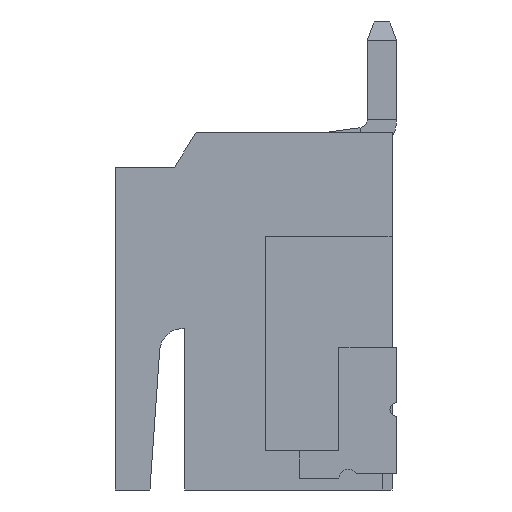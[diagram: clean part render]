
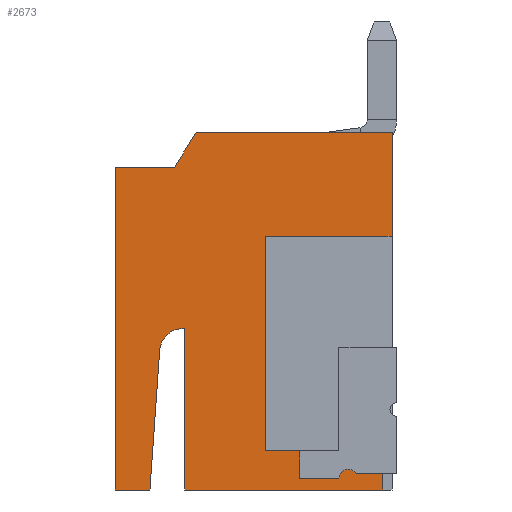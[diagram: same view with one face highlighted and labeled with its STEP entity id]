
A CAD part, left-side view. The second image highlights one B-rep face of the part: STEP entity #2673.
In plain terms, the highlighted planar face has unit normal (-1, 0, 0).
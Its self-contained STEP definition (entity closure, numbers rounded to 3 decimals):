
#42 = DIRECTION ( 'NONE',  ( 0., 0., 1. ) ) ;
#72 = DIRECTION ( 'NONE',  ( 0., 0., -1. ) ) ;
#179 = EDGE_CURVE ( 'NONE', #2912, #4283, #1416, .T. ) ;
#268 = LINE ( 'NONE', #2807, #2163 ) ;
#281 = CARTESIAN_POINT ( 'NONE',  ( -6.25, -3.1, 3.875 ) ) ;
#428 = DIRECTION ( 'NONE',  ( 0., 0., 1. ) ) ;
#491 = CARTESIAN_POINT ( 'NONE',  ( -6.25, 1.619, 3.125 ) ) ;
#529 = CARTESIAN_POINT ( 'NONE',  ( -6.25, -2.9, 3.875 ) ) ;
#533 = CARTESIAN_POINT ( 'NONE',  ( -6.25, -2.9, -3.525 ) ) ;
#568 = VECTOR ( 'NONE', #6327, 1000. ) ;
#625 = LINE ( 'NONE', #2637, #4047 ) ;
#631 = CARTESIAN_POINT ( 'NONE',  ( -6.25, 1.87, 0.131 ) ) ;
#666 = ORIENTED_EDGE ( 'NONE', *, *, #1401, .T. ) ;
#697 = EDGE_CURVE ( 'NONE', #4283, #6378, #1847, .T. ) ;
#701 = CARTESIAN_POINT ( 'NONE',  ( -6.25, -2.15, -3.625 ) ) ;
#812 = EDGE_CURVE ( 'NONE', #3117, #1203, #4040, .T. ) ;
#851 = DIRECTION ( 'NONE',  ( 0., 1., 0. ) ) ;
#862 = AXIS2_PLACEMENT_3D ( 'NONE', #4257, #6275, #2281 ) ;
#914 = ORIENTED_EDGE ( 'NONE', *, *, #1289, .T. ) ;
#956 = DIRECTION ( 'NONE',  ( 0., 1., 0. ) ) ;
#1022 = CARTESIAN_POINT ( 'NONE',  ( -6.25, -0.35, 1.625 ) ) ;
#1098 = CARTESIAN_POINT ( 'NONE',  ( -6.25, -2.323, -3.525 ) ) ;
#1147 = ORIENTED_EDGE ( 'NONE', *, *, #5128, .T. ) ;
#1203 = VERTEX_POINT ( 'NONE', #2487 ) ;
#1289 = EDGE_CURVE ( 'NONE', #4978, #3504, #3168, .T. ) ;
#1334 = CARTESIAN_POINT ( 'NONE',  ( -6.25, -0.35, 1.625 ) ) ;
#1401 = EDGE_CURVE ( 'NONE', #1934, #2912, #5885, .T. ) ;
#1416 = LINE ( 'NONE', #2936, #2177 ) ;
#1480 = CARTESIAN_POINT ( 'NONE',  ( -6.25, 1.439, -0.873 ) ) ;
#1496 = ORIENTED_EDGE ( 'NONE', *, *, #6158, .F. ) ;
#1528 = VECTOR ( 'NONE', #956, 1000. ) ;
#1649 = LINE ( 'NONE', #529, #2906 ) ;
#1666 = ORIENTED_EDGE ( 'NONE', *, *, #3754, .F. ) ;
#1847 = LINE ( 'NONE', #3853, #3435 ) ;
#1856 = CARTESIAN_POINT ( 'NONE',  ( -6.25, -0.35, -3.025 ) ) ;
#1871 = DIRECTION ( 'NONE',  ( 0., 0., -1. ) ) ;
#1874 = VERTEX_POINT ( 'NONE', #2864 ) ;
#1908 = CARTESIAN_POINT ( 'NONE',  ( -6.25, 2.15, -3.875 ) ) ;
#1934 = VERTEX_POINT ( 'NONE', #3322 ) ;
#1966 = CARTESIAN_POINT ( 'NONE',  ( -6.25, 1.4, -3.875 ) ) ;
#2133 = LINE ( 'NONE', #2265, #3410 ) ;
#2143 = CARTESIAN_POINT ( 'NONE',  ( -6.25, -1.95, -3.625 ) ) ;
#2163 = VECTOR ( 'NONE', #851, 1000. ) ;
#2177 = VECTOR ( 'NONE', #2342, 1000. ) ;
#2216 = DIRECTION ( 'NONE',  ( 0., 0., -1. ) ) ;
#2247 = PLANE ( 'NONE',  #862 ) ;
#2265 = CARTESIAN_POINT ( 'NONE',  ( -6.25, 1.4, 0. ) ) ;
#2281 = DIRECTION ( 'NONE',  ( 0., 0., -1. ) ) ;
#2288 = VECTOR ( 'NONE', #4508, 1000. ) ;
#2342 = DIRECTION ( 'NONE',  ( 0., -1., 0. ) ) ;
#2443 = CARTESIAN_POINT ( 'NONE',  ( -6.25, -2.9, -3.875 ) ) ;
#2474 = VECTOR ( 'NONE', #4161, 1000. ) ;
#2487 = CARTESIAN_POINT ( 'NONE',  ( -6.25, 1.15, 3.875 ) ) ;
#2637 = CARTESIAN_POINT ( 'NONE',  ( -6.25, 1.15, 3.875 ) ) ;
#2673 = ADVANCED_FACE ( 'NONE', ( #2741 ), #2247, .F. ) ;
#2679 = ORIENTED_EDGE ( 'NONE', *, *, #2937, .T. ) ;
#2693 = CIRCLE ( 'NONE', #4911, 0.2 ) ;
#2711 = DIRECTION ( 'NONE',  ( -1., 0., 0. ) ) ;
#2733 = CIRCLE ( 'NONE', #3457, 0.5 ) ;
#2741 = FACE_OUTER_BOUND ( 'NONE', #5272, .T. ) ;
#2761 = CARTESIAN_POINT ( 'NONE',  ( -6.25, -3.1, 1.625 ) ) ;
#2807 = CARTESIAN_POINT ( 'NONE',  ( -6.25, -2.9, -3.875 ) ) ;
#2821 = DIRECTION ( 'NONE',  ( 0., -1., 0. ) ) ;
#2848 = ORIENTED_EDGE ( 'NONE', *, *, #812, .F. ) ;
#2864 = CARTESIAN_POINT ( 'NONE',  ( -6.25, 1.938, -0.839 ) ) ;
#2906 = VECTOR ( 'NONE', #6130, 1000. ) ;
#2912 = VERTEX_POINT ( 'NONE', #1022 ) ;
#2936 = CARTESIAN_POINT ( 'NONE',  ( -6.25, -2.9, 1.625 ) ) ;
#2937 = EDGE_CURVE ( 'NONE', #1874, #6040, #2733, .T. ) ;
#2954 = VERTEX_POINT ( 'NONE', #3085 ) ;
#2974 = CARTESIAN_POINT ( 'NONE',  ( -6.25, 1.4, -0.375 ) ) ;
#3073 = ORIENTED_EDGE ( 'NONE', *, *, #4205, .F. ) ;
#3085 = CARTESIAN_POINT ( 'NONE',  ( -6.25, 2.9, 3.125 ) ) ;
#3087 = DIRECTION ( 'NONE',  ( 0., -1., 0. ) ) ;
#3117 = VERTEX_POINT ( 'NONE', #4441 ) ;
#3130 = CARTESIAN_POINT ( 'NONE',  ( -6.25, 2.9, -3.875 ) ) ;
#3132 = VERTEX_POINT ( 'NONE', #1908 ) ;
#3168 = LINE ( 'NONE', #1098, #4431 ) ;
#3199 = ORIENTED_EDGE ( 'NONE', *, *, #5900, .F. ) ;
#3243 = ORIENTED_EDGE ( 'NONE', *, *, #5388, .F. ) ;
#3322 = CARTESIAN_POINT ( 'NONE',  ( -6.25, -0.35, -3.025 ) ) ;
#3410 = VECTOR ( 'NONE', #1871, 1000. ) ;
#3422 = VECTOR ( 'NONE', #42, 1000. ) ;
#3435 = VECTOR ( 'NONE', #428, 1000. ) ;
#3457 = AXIS2_PLACEMENT_3D ( 'NONE', #1480, #3486, #72 ) ;
#3486 = DIRECTION ( 'NONE',  ( 1., 0., 0. ) ) ;
#3504 = VERTEX_POINT ( 'NONE', #5168 ) ;
#3531 = ORIENTED_EDGE ( 'NONE', *, *, #179, .T. ) ;
#3579 = VECTOR ( 'NONE', #4302, 1000. ) ;
#3591 = CARTESIAN_POINT ( 'NONE',  ( -6.25, -1.1, -3.025 ) ) ;
#3684 = VERTEX_POINT ( 'NONE', #4045 ) ;
#3695 = CARTESIAN_POINT ( 'NONE',  ( -6.25, 2.9, -3.875 ) ) ;
#3754 = EDGE_CURVE ( 'NONE', #3132, #6255, #268, .T. ) ;
#3849 = VECTOR ( 'NONE', #4857, 1000. ) ;
#3853 = CARTESIAN_POINT ( 'NONE',  ( -6.25, -3.1, 3.875 ) ) ;
#3933 = ORIENTED_EDGE ( 'NONE', *, *, #4157, .T. ) ;
#4040 = LINE ( 'NONE', #491, #2288 ) ;
#4045 = CARTESIAN_POINT ( 'NONE',  ( -6.25, -1.1, -3.625 ) ) ;
#4047 = VECTOR ( 'NONE', #3087, 1000. ) ;
#4157 = EDGE_CURVE ( 'NONE', #6040, #5623, #2133, .T. ) ;
#4161 = DIRECTION ( 'NONE',  ( 0., -0.07, 0.998 ) ) ;
#4194 = LINE ( 'NONE', #3130, #3422 ) ;
#4205 = EDGE_CURVE ( 'NONE', #4726, #5623, #6260, .T. ) ;
#4257 = CARTESIAN_POINT ( 'NONE',  ( -6.25, 0., 0. ) ) ;
#4283 = VERTEX_POINT ( 'NONE', #2761 ) ;
#4302 = DIRECTION ( 'NONE',  ( 0., 0., 1. ) ) ;
#4431 = VECTOR ( 'NONE', #6141, 1000. ) ;
#4441 = CARTESIAN_POINT ( 'NONE',  ( -6.25, 1.619, 3.125 ) ) ;
#4508 = DIRECTION ( 'NONE',  ( 0., -0.53, 0.848 ) ) ;
#4726 = VERTEX_POINT ( 'NONE', #2443 ) ;
#4857 = DIRECTION ( 'NONE',  ( 0., 0., 1. ) ) ;
#4911 = AXIS2_PLACEMENT_3D ( 'NONE', #701, #2711, #2216 ) ;
#4978 = VERTEX_POINT ( 'NONE', #533 ) ;
#5019 = LINE ( 'NONE', #1856, #5228 ) ;
#5041 = ORIENTED_EDGE ( 'NONE', *, *, #697, .T. ) ;
#5087 = EDGE_CURVE ( 'NONE', #3684, #6299, #5256, .T. ) ;
#5105 = ORIENTED_EDGE ( 'NONE', *, *, #5087, .T. ) ;
#5128 = EDGE_CURVE ( 'NONE', #3504, #5326, #2693, .T. ) ;
#5153 = LINE ( 'NONE', #631, #2474 ) ;
#5168 = CARTESIAN_POINT ( 'NONE',  ( -6.25, -2.323, -3.525 ) ) ;
#5220 = EDGE_CURVE ( 'NONE', #5326, #3684, #5447, .T. ) ;
#5228 = VECTOR ( 'NONE', #5383, 1000. ) ;
#5256 = LINE ( 'NONE', #5814, #3849 ) ;
#5272 = EDGE_LOOP ( 'NONE', ( #2679, #3933, #3073, #3243, #914, #1147, #6092, #5105, #6409, #666, #3531, #5041, #6064, #2848, #3199, #1496, #1666, #5760 ) ) ;
#5294 = EDGE_CURVE ( 'NONE', #6299, #1934, #5019, .T. ) ;
#5326 = VERTEX_POINT ( 'NONE', #2143 ) ;
#5331 = LINE ( 'NONE', #5789, #5629 ) ;
#5383 = DIRECTION ( 'NONE',  ( 0., 1., 0. ) ) ;
#5388 = EDGE_CURVE ( 'NONE', #4978, #4726, #1649, .T. ) ;
#5416 = EDGE_CURVE ( 'NONE', #1203, #6378, #625, .T. ) ;
#5447 = LINE ( 'NONE', #6467, #1528 ) ;
#5623 = VERTEX_POINT ( 'NONE', #1966 ) ;
#5629 = VECTOR ( 'NONE', #2821, 1000. ) ;
#5760 = ORIENTED_EDGE ( 'NONE', *, *, #6247, .T. ) ;
#5789 = CARTESIAN_POINT ( 'NONE',  ( -6.25, 2.9, 3.125 ) ) ;
#5814 = CARTESIAN_POINT ( 'NONE',  ( -6.25, -1.1, -0.775 ) ) ;
#5885 = LINE ( 'NONE', #1334, #3579 ) ;
#5900 = EDGE_CURVE ( 'NONE', #2954, #3117, #5331, .T. ) ;
#6040 = VERTEX_POINT ( 'NONE', #2974 ) ;
#6064 = ORIENTED_EDGE ( 'NONE', *, *, #5416, .F. ) ;
#6092 = ORIENTED_EDGE ( 'NONE', *, *, #5220, .T. ) ;
#6130 = DIRECTION ( 'NONE',  ( 0., 0., -1. ) ) ;
#6141 = DIRECTION ( 'NONE',  ( 0., 1., 0. ) ) ;
#6158 = EDGE_CURVE ( 'NONE', #6255, #2954, #4194, .T. ) ;
#6247 = EDGE_CURVE ( 'NONE', #3132, #1874, #5153, .T. ) ;
#6255 = VERTEX_POINT ( 'NONE', #3695 ) ;
#6260 = LINE ( 'NONE', #6392, #568 ) ;
#6275 = DIRECTION ( 'NONE',  ( 1., 0., 0. ) ) ;
#6299 = VERTEX_POINT ( 'NONE', #3591 ) ;
#6327 = DIRECTION ( 'NONE',  ( 0., 1., 0. ) ) ;
#6378 = VERTEX_POINT ( 'NONE', #281 ) ;
#6392 = CARTESIAN_POINT ( 'NONE',  ( -6.25, -2.9, -3.875 ) ) ;
#6409 = ORIENTED_EDGE ( 'NONE', *, *, #5294, .T. ) ;
#6467 = CARTESIAN_POINT ( 'NONE',  ( -6.25, -1.1, -3.625 ) ) ;
